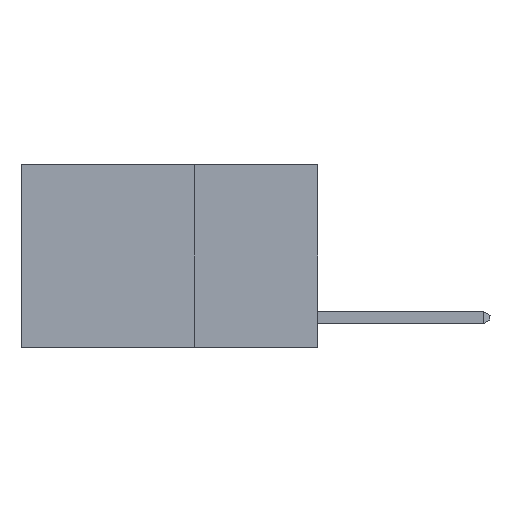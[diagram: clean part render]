
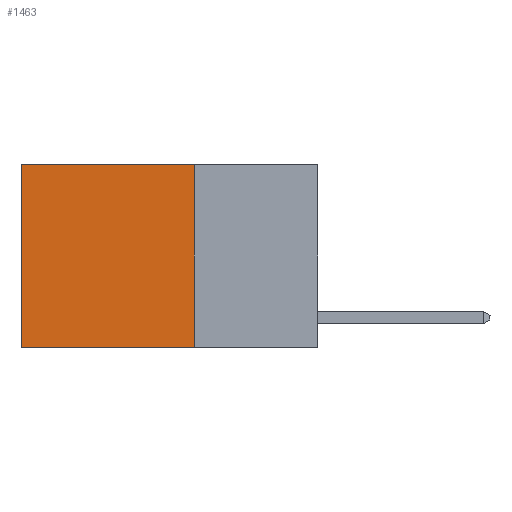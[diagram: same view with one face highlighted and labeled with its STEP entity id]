
A CAD part, left-side view. The second image highlights one B-rep face of the part: STEP entity #1463.
In plain terms, the highlighted planar face has unit normal (-1, 0, 0).
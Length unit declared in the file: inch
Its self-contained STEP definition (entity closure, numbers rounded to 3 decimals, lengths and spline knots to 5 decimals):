
#248 = ORIENTED_EDGE ( 'NONE', *, *, #10508, .T. ) ;
#453 = VECTOR ( 'NONE', #3273, 39.37008 ) ;
#837 = VERTEX_POINT ( 'NONE', #4437 ) ;
#1386 = VERTEX_POINT ( 'NONE', #10019 ) ;
#1449 = AXIS2_PLACEMENT_3D ( 'NONE', #1656, #7024, #9295 ) ;
#1463 = ADVANCED_FACE ( 'NONE', ( #10295 ), #6889, .F. ) ;
#1656 = CARTESIAN_POINT ( 'NONE',  ( 0.2625, 0.25, 0. ) ) ;
#1730 = LINE ( 'NONE', #6022, #453 ) ;
#1810 = DIRECTION ( 'NONE',  ( 0., 1., 0. ) ) ;
#2007 = DIRECTION ( 'NONE',  ( 0., 0., -1. ) ) ;
#2090 = VECTOR ( 'NONE', #1810, 39.37008 ) ;
#2622 = EDGE_CURVE ( 'NONE', #6890, #837, #10431, .T. ) ;
#2753 = LINE ( 'NONE', #7072, #10042 ) ;
#3273 = DIRECTION ( 'NONE',  ( 0., 0., -1. ) ) ;
#4341 = CARTESIAN_POINT ( 'NONE',  ( 0.2625, 0.25, 0. ) ) ;
#4437 = CARTESIAN_POINT ( 'NONE',  ( 0.2625, 0.6, -0.37 ) ) ;
#4456 = CARTESIAN_POINT ( 'NONE',  ( 0.2625, 0.6, 0. ) ) ;
#4779 = EDGE_LOOP ( 'NONE', ( #7881, #11255, #7607, #248 ) ) ;
#5796 = EDGE_CURVE ( 'NONE', #10668, #1386, #1730, .T. ) ;
#6022 = CARTESIAN_POINT ( 'NONE',  ( 0.2625, 0.25, 0. ) ) ;
#6889 = PLANE ( 'NONE',  #1449 ) ;
#6890 = VERTEX_POINT ( 'NONE', #4456 ) ;
#7024 = DIRECTION ( 'NONE',  ( 1., 0., 0. ) ) ;
#7072 = CARTESIAN_POINT ( 'NONE',  ( 0.2625, 0.25, -0.37 ) ) ;
#7607 = ORIENTED_EDGE ( 'NONE', *, *, #5796, .F. ) ;
#7881 = ORIENTED_EDGE ( 'NONE', *, *, #2622, .T. ) ;
#7912 = VECTOR ( 'NONE', #2007, 39.37008 ) ;
#9295 = DIRECTION ( 'NONE',  ( 0., 0., -1. ) ) ;
#10019 = CARTESIAN_POINT ( 'NONE',  ( 0.2625, 0.25, -0.37 ) ) ;
#10042 = VECTOR ( 'NONE', #10757, 39.37008 ) ;
#10295 = FACE_OUTER_BOUND ( 'NONE', #4779, .T. ) ;
#10431 = LINE ( 'NONE', #11621, #7912 ) ;
#10508 = EDGE_CURVE ( 'NONE', #10668, #6890, #12683, .T. ) ;
#10668 = VERTEX_POINT ( 'NONE', #4341 ) ;
#10757 = DIRECTION ( 'NONE',  ( 0., 1., 0. ) ) ;
#11255 = ORIENTED_EDGE ( 'NONE', *, *, #13624, .F. ) ;
#11621 = CARTESIAN_POINT ( 'NONE',  ( 0.2625, 0.6, 0. ) ) ;
#12683 = LINE ( 'NONE', #13731, #2090 ) ;
#13624 = EDGE_CURVE ( 'NONE', #1386, #837, #2753, .T. ) ;
#13731 = CARTESIAN_POINT ( 'NONE',  ( 0.2625, 0.25, 0. ) ) ;
